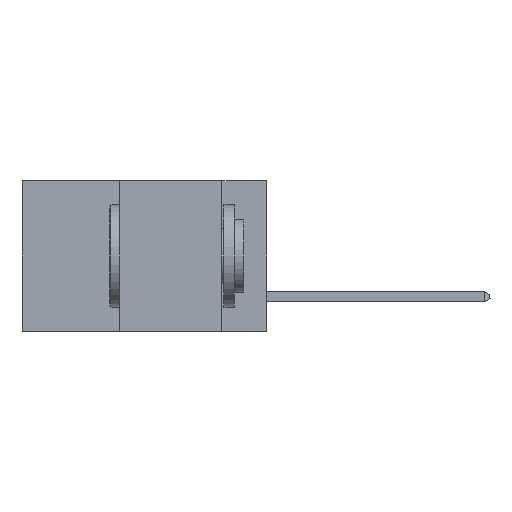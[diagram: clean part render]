
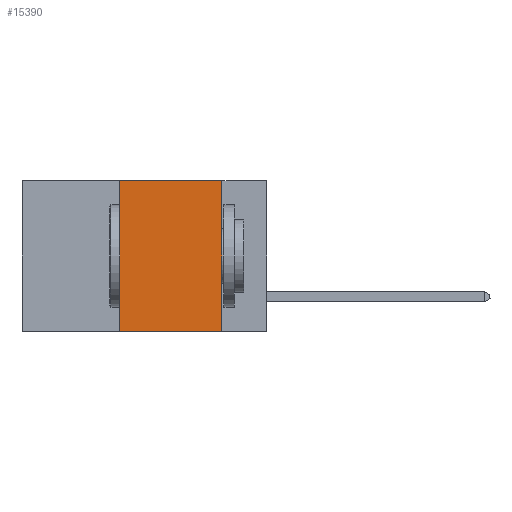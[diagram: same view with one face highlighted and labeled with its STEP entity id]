
A CAD part, left-side view. The second image highlights one B-rep face of the part: STEP entity #15390.
In plain terms, the highlighted planar face has unit normal (-1, 0, 0).
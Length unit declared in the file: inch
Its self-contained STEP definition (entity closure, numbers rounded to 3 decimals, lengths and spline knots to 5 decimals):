
#644 = CARTESIAN_POINT ( 'NONE',  ( 0., 0.6, -0.37 ) ) ;
#1541 = FACE_OUTER_BOUND ( 'NONE', #31366, .T. ) ;
#2067 = EDGE_CURVE ( 'NONE', #27524, #28765, #12093, .T. ) ;
#4392 = ORIENTED_EDGE ( 'NONE', *, *, #2067, .T. ) ;
#4826 = VECTOR ( 'NONE', #11508, 39.37008 ) ;
#4985 = VECTOR ( 'NONE', #10050, 39.37008 ) ;
#5051 = VECTOR ( 'NONE', #20401, 39.37008 ) ;
#6092 = CARTESIAN_POINT ( 'NONE',  ( 0., 0.11, 0. ) ) ;
#8671 = ORIENTED_EDGE ( 'NONE', *, *, #23185, .F. ) ;
#10050 = DIRECTION ( 'NONE',  ( 0., 0., 1. ) ) ;
#10175 = CARTESIAN_POINT ( 'NONE',  ( 0., 0.11, -0.37 ) ) ;
#10251 = AXIS2_PLACEMENT_3D ( 'NONE', #29236, #26251, #16680 ) ;
#11508 = DIRECTION ( 'NONE',  ( 0., 0., -1. ) ) ;
#12093 = LINE ( 'NONE', #644, #5051 ) ;
#15328 = LINE ( 'NONE', #23228, #4985 ) ;
#15390 = ADVANCED_FACE ( 'NONE', ( #1541 ), #21140, .F. ) ;
#16680 = DIRECTION ( 'NONE',  ( 0., 0., -1. ) ) ;
#19275 = ORIENTED_EDGE ( 'NONE', *, *, #20872, .F. ) ;
#20109 = CARTESIAN_POINT ( 'NONE',  ( 0., 0.36, -0.37 ) ) ;
#20401 = DIRECTION ( 'NONE',  ( 0., -1., 0. ) ) ;
#20872 = EDGE_CURVE ( 'NONE', #29117, #28765, #23902, .T. ) ;
#21140 = PLANE ( 'NONE',  #10251 ) ;
#21622 = EDGE_CURVE ( 'NONE', #27524, #30043, #15328, .T. ) ;
#23185 = EDGE_CURVE ( 'NONE', #30043, #29117, #32990, .T. ) ;
#23228 = CARTESIAN_POINT ( 'NONE',  ( 0., 0.36, 0. ) ) ;
#23811 = DIRECTION ( 'NONE',  ( 0., -1., 0. ) ) ;
#23902 = LINE ( 'NONE', #24957, #4826 ) ;
#24957 = CARTESIAN_POINT ( 'NONE',  ( 0., 0.11, 0. ) ) ;
#26251 = DIRECTION ( 'NONE',  ( 1., 0., 0. ) ) ;
#27524 = VERTEX_POINT ( 'NONE', #20109 ) ;
#28765 = VERTEX_POINT ( 'NONE', #10175 ) ;
#29117 = VERTEX_POINT ( 'NONE', #6092 ) ;
#29145 = CARTESIAN_POINT ( 'NONE',  ( 0., 0.6, 0. ) ) ;
#29236 = CARTESIAN_POINT ( 'NONE',  ( 0., 0.6, 0. ) ) ;
#30043 = VERTEX_POINT ( 'NONE', #31427 ) ;
#31366 = EDGE_LOOP ( 'NONE', ( #19275, #8671, #32574, #4392 ) ) ;
#31427 = CARTESIAN_POINT ( 'NONE',  ( 0., 0.36, 0. ) ) ;
#31751 = VECTOR ( 'NONE', #23811, 39.37008 ) ;
#32574 = ORIENTED_EDGE ( 'NONE', *, *, #21622, .F. ) ;
#32990 = LINE ( 'NONE', #29145, #31751 ) ;
